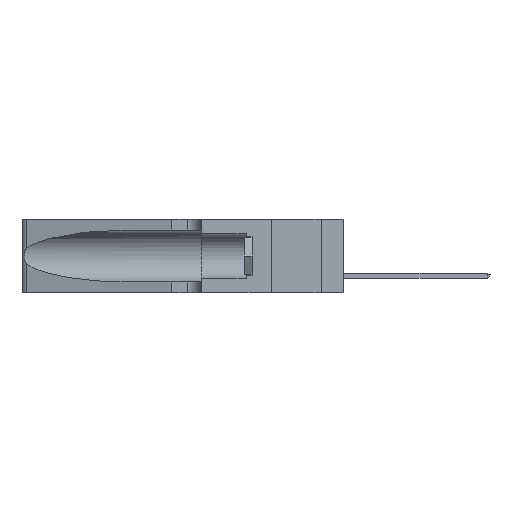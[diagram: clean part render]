
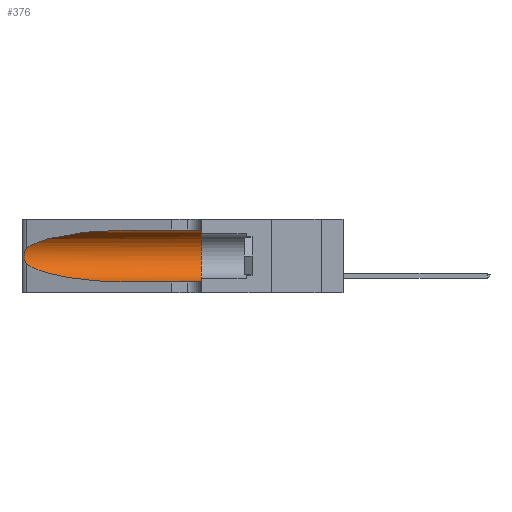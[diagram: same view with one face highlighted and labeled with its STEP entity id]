
A CAD part, left-side view. The second image highlights one B-rep face of the part: STEP entity #376.
In plain terms, the highlighted cylindrical face has radius 3.308 mm (diameter 6.617 mm), a partial arc.
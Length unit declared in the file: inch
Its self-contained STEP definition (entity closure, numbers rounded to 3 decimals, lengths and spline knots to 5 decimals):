
#376 = ADVANCED_FACE ( 'NONE', ( #15906 ), #19862, .F. ) ;
#1056 = EDGE_CURVE ( 'NONE', #12062, #26775, #25892, .T. ) ;
#1414 = CARTESIAN_POINT ( 'NONE',  ( 0.1305, 1.61858, 0.185 ) ) ;
#1641 = DIRECTION ( 'NONE',  ( 0., 0., 1. ) ) ;
#1822 = EDGE_LOOP ( 'NONE', ( #24559, #20884, #5810, #10615, #25988, #15130 ) ) ;
#1895 = CARTESIAN_POINT ( 'NONE',  ( 0.1305, 0.72297, 0.05475 ) ) ;
#2195 = CARTESIAN_POINT ( 'NONE',  ( 0.1305, 1.61858, 0.05475 ) ) ;
#2304 = EDGE_CURVE ( 'NONE', #22984, #6280, #2570, .T. ) ;
#2390 = CARTESIAN_POINT ( 'NONE',  ( 0.18966, 0.96281, 0.31525 ) ) ;
#2453 = LINE ( 'NONE', #11097, #26103 ) ;
#2570 = CIRCLE ( 'NONE', #13872, 0.13025 ) ;
#2852 = VERTEX_POINT ( 'NONE', #11820 ) ;
#3589 = CARTESIAN_POINT ( 'NONE',  ( 0.1305, 0.35, 0.31525 ) ) ;
#4681 = CARTESIAN_POINT ( 'NONE',  ( 0.25487, 1.22718, 0.22369 ) ) ;
#5045 = EDGE_CURVE ( 'NONE', #24068, #12062, #20602, .T. ) ;
#5810 = ORIENTED_EDGE ( 'NONE', *, *, #9718, .T. ) ;
#6280 = VERTEX_POINT ( 'NONE', #10479 ) ;
#7572 = CARTESIAN_POINT ( 'NONE',  ( 0.25854, 1.2359, 0.20912 ) ) ;
#7724 =( BOUNDED_CURVE ( )  B_SPLINE_CURVE ( 3, ( #19923, #24126, #10796, #1895 ),
 .UNSPECIFIED., .F., .T. ) 
 B_SPLINE_CURVE_WITH_KNOTS ( ( 4, 4 ),
 ( 3.44316, 4.71239 ),
 .UNSPECIFIED. ) 
 CURVE ( )  GEOMETRIC_REPRESENTATION_ITEM ( )  RATIONAL_B_SPLINE_CURVE ( ( 1., 0.87, 0.87, 1. ) ) 
 REPRESENTATION_ITEM ( '' )  );
#8732 = CARTESIAN_POINT ( 'NONE',  ( 0.1305, 0.35, 0.185 ) ) ;
#8897 = DIRECTION ( 'NONE',  ( 0., -1., 0. ) ) ;
#9661 = CARTESIAN_POINT ( 'NONE',  ( 0.25639, 1.23184, 0.21858 ) ) ;
#9718 = EDGE_CURVE ( 'NONE', #26775, #2852, #7724, .T. ) ;
#10479 = CARTESIAN_POINT ( 'NONE',  ( 0.1305, 0.35, 0.05475 ) ) ;
#10571 = CARTESIAN_POINT ( 'NONE',  ( 0.25487, 1.22718, 0.14631 ) ) ;
#10615 = ORIENTED_EDGE ( 'NONE', *, *, #23754, .T. ) ;
#10796 = CARTESIAN_POINT ( 'NONE',  ( 0.18966, 0.96281, 0.05475 ) ) ;
#11097 = CARTESIAN_POINT ( 'NONE',  ( 0.1305, 1.61858, 0.31525 ) ) ;
#11375 = CARTESIAN_POINT ( 'NONE',  ( 0.2373, 1.15595, 0.28018 ) ) ;
#11549 = CARTESIAN_POINT ( 'NONE',  ( 0.25639, 1.23186, 0.15144 ) ) ;
#11820 = CARTESIAN_POINT ( 'NONE',  ( 0.1305, 0.72297, 0.05475 ) ) ;
#12062 = VERTEX_POINT ( 'NONE', #14517 ) ;
#12063 = CARTESIAN_POINT ( 'NONE',  ( 0.26018, 1.23835, 0.19895 ) ) ;
#12388 = AXIS2_PLACEMENT_3D ( 'NONE', #1414, #8897, #24847 ) ;
#13397 = DIRECTION ( 'NONE',  ( 0., -1., 0. ) ) ;
#13586 = CARTESIAN_POINT ( 'NONE',  ( 0.26017, 1.23833, 0.17102 ) ) ;
#13841 = CARTESIAN_POINT ( 'NONE',  ( 0.25487, 1.22718, 0.14631 ) ) ;
#13872 = AXIS2_PLACEMENT_3D ( 'NONE', #8732, #29069, #1641 ) ;
#14262 = CARTESIAN_POINT ( 'NONE',  ( 0.25787, 1.23484, 0.2124 ) ) ;
#14517 = CARTESIAN_POINT ( 'NONE',  ( 0.25487, 1.22718, 0.22369 ) ) ;
#14898 = CARTESIAN_POINT ( 'NONE',  ( 0.26075, 1.23896, 0.178 ) ) ;
#15130 = ORIENTED_EDGE ( 'NONE', *, *, #18477, .F. ) ;
#15906 = FACE_OUTER_BOUND ( 'NONE', #1822, .T. ) ;
#16304 = CARTESIAN_POINT ( 'NONE',  ( 0.1305, 0.72297, 0.31525 ) ) ;
#17887 = LINE ( 'NONE', #2195, #29345 ) ;
#18477 = EDGE_CURVE ( 'NONE', #24068, #22984, #2453, .T. ) ;
#18730 = CARTESIAN_POINT ( 'NONE',  ( 0.25487, 1.22718, 0.22369 ) ) ;
#18980 = CARTESIAN_POINT ( 'NONE',  ( 0.26075, 1.23896, 0.19203 ) ) ;
#19862 = CYLINDRICAL_SURFACE ( 'NONE', #12388, 0.13025 ) ;
#19923 = CARTESIAN_POINT ( 'NONE',  ( 0.25487, 1.22718, 0.14631 ) ) ;
#20602 =( BOUNDED_CURVE ( )  B_SPLINE_CURVE ( 3, ( #16304, #2390, #11375, #4681 ),
 .UNSPECIFIED., .F., .F. ) 
 B_SPLINE_CURVE_WITH_KNOTS ( ( 4, 4 ),
 ( 1.5708, 2.84003 ),
 .UNSPECIFIED. ) 
 CURVE ( )  GEOMETRIC_REPRESENTATION_ITEM ( )  RATIONAL_B_SPLINE_CURVE ( ( 1., 0.87, 0.87, 1. ) ) 
 REPRESENTATION_ITEM ( '' )  );
#20884 = ORIENTED_EDGE ( 'NONE', *, *, #1056, .T. ) ;
#22984 = VERTEX_POINT ( 'NONE', #3589 ) ;
#23754 = EDGE_CURVE ( 'NONE', #2852, #6280, #17887, .T. ) ;
#24068 = VERTEX_POINT ( 'NONE', #27332 ) ;
#24094 = CARTESIAN_POINT ( 'NONE',  ( 0.25555, 1.22994, 0.2215 ) ) ;
#24126 = CARTESIAN_POINT ( 'NONE',  ( 0.2373, 1.15595, 0.08982 ) ) ;
#24559 = ORIENTED_EDGE ( 'NONE', *, *, #5045, .T. ) ;
#24847 = DIRECTION ( 'NONE',  ( 0., 0., -1. ) ) ;
#25188 = CARTESIAN_POINT ( 'NONE',  ( 0.25555, 1.22993, 0.14849 ) ) ;
#25892 = B_SPLINE_CURVE_WITH_KNOTS ( 'NONE', 3,
 ( #18730, #24094, #9661, #14262, #7572, #12063, #18980, #14898, #13586, #27396, #29577, #11549, #25188, #13841 ),
 .UNSPECIFIED., .F., .F.,
 ( 4, 2, 2, 2, 2, 2, 4 ),
 ( 0., 0.00027, 0.00053, 0.00107, 0.0016, 0.00187, 0.00214 ),
 .UNSPECIFIED. ) ;
#25988 = ORIENTED_EDGE ( 'NONE', *, *, #2304, .F. ) ;
#26103 = VECTOR ( 'NONE', #13397, 39.37008 ) ;
#26775 = VERTEX_POINT ( 'NONE', #10571 ) ;
#27332 = CARTESIAN_POINT ( 'NONE',  ( 0.1305, 0.72297, 0.31525 ) ) ;
#27396 = CARTESIAN_POINT ( 'NONE',  ( 0.25856, 1.23593, 0.16098 ) ) ;
#29069 = DIRECTION ( 'NONE',  ( 0., 1., 0. ) ) ;
#29345 = VECTOR ( 'NONE', #29392, 39.37008 ) ;
#29392 = DIRECTION ( 'NONE',  ( 0., -1., 0. ) ) ;
#29577 = CARTESIAN_POINT ( 'NONE',  ( 0.25789, 1.23486, 0.15765 ) ) ;
